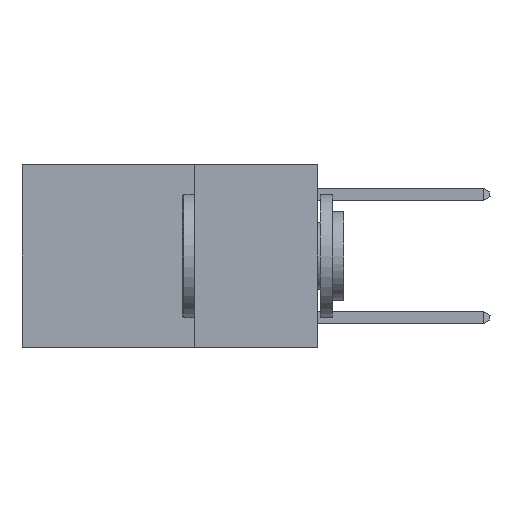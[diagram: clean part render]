
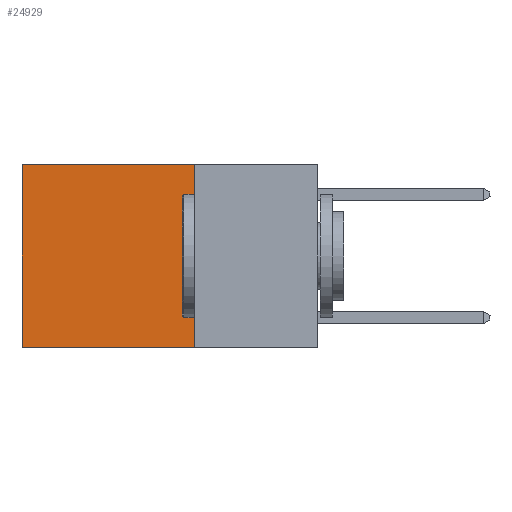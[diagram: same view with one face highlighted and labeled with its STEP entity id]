
A CAD part, left-side view. The second image highlights one B-rep face of the part: STEP entity #24929.
In plain terms, the highlighted planar face has unit normal (-1, 0, 0).
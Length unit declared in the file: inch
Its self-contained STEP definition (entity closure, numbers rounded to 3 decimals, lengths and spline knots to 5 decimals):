
#1169 = CARTESIAN_POINT ( 'NONE',  ( 0.2625, 0.25, -0.37 ) ) ;
#2375 = CARTESIAN_POINT ( 'NONE',  ( 0.2625, 0.6, 0. ) ) ;
#2549 = LINE ( 'NONE', #26830, #11363 ) ;
#3791 = DIRECTION ( 'NONE',  ( 0., 1., 0. ) ) ;
#3831 = EDGE_CURVE ( 'NONE', #21068, #22436, #2549, .T. ) ;
#3888 = ORIENTED_EDGE ( 'NONE', *, *, #3831, .F. ) ;
#4287 = EDGE_LOOP ( 'NONE', ( #21799, #28742, #3888, #22203 ) ) ;
#5786 = FACE_OUTER_BOUND ( 'NONE', #4287, .T. ) ;
#6304 = EDGE_CURVE ( 'NONE', #22436, #11542, #26907, .T. ) ;
#8492 = CARTESIAN_POINT ( 'NONE',  ( 0.2625, 0.6, -0.37 ) ) ;
#8498 = VECTOR ( 'NONE', #29847, 39.37008 ) ;
#10286 = DIRECTION ( 'NONE',  ( 1., 0., 0. ) ) ;
#10897 = EDGE_CURVE ( 'NONE', #21068, #19864, #11198, .T. ) ;
#11114 = CARTESIAN_POINT ( 'NONE',  ( 0.2625, 0.25, -0.37 ) ) ;
#11198 = LINE ( 'NONE', #18161, #18607 ) ;
#11363 = VECTOR ( 'NONE', #28298, 39.37008 ) ;
#11542 = VERTEX_POINT ( 'NONE', #8492 ) ;
#13264 = CARTESIAN_POINT ( 'NONE',  ( 0.2625, 0.6, 0. ) ) ;
#17571 = AXIS2_PLACEMENT_3D ( 'NONE', #22087, #10286, #19746 ) ;
#17903 = LINE ( 'NONE', #13264, #8498 ) ;
#18161 = CARTESIAN_POINT ( 'NONE',  ( 0.2625, 0.25, 0. ) ) ;
#18607 = VECTOR ( 'NONE', #20339, 39.37008 ) ;
#19746 = DIRECTION ( 'NONE',  ( 0., 0., -1. ) ) ;
#19760 = EDGE_CURVE ( 'NONE', #19864, #11542, #17903, .T. ) ;
#19864 = VERTEX_POINT ( 'NONE', #2375 ) ;
#20202 = PLANE ( 'NONE',  #17571 ) ;
#20339 = DIRECTION ( 'NONE',  ( 0., 1., 0. ) ) ;
#20778 = VECTOR ( 'NONE', #3791, 39.37008 ) ;
#21068 = VERTEX_POINT ( 'NONE', #22702 ) ;
#21799 = ORIENTED_EDGE ( 'NONE', *, *, #19760, .T. ) ;
#22087 = CARTESIAN_POINT ( 'NONE',  ( 0.2625, 0.25, 0. ) ) ;
#22203 = ORIENTED_EDGE ( 'NONE', *, *, #10897, .T. ) ;
#22436 = VERTEX_POINT ( 'NONE', #11114 ) ;
#22702 = CARTESIAN_POINT ( 'NONE',  ( 0.2625, 0.25, 0. ) ) ;
#24929 = ADVANCED_FACE ( 'NONE', ( #5786 ), #20202, .F. ) ;
#26830 = CARTESIAN_POINT ( 'NONE',  ( 0.2625, 0.25, 0. ) ) ;
#26907 = LINE ( 'NONE', #1169, #20778 ) ;
#28298 = DIRECTION ( 'NONE',  ( 0., 0., -1. ) ) ;
#28742 = ORIENTED_EDGE ( 'NONE', *, *, #6304, .F. ) ;
#29847 = DIRECTION ( 'NONE',  ( 0., 0., -1. ) ) ;
